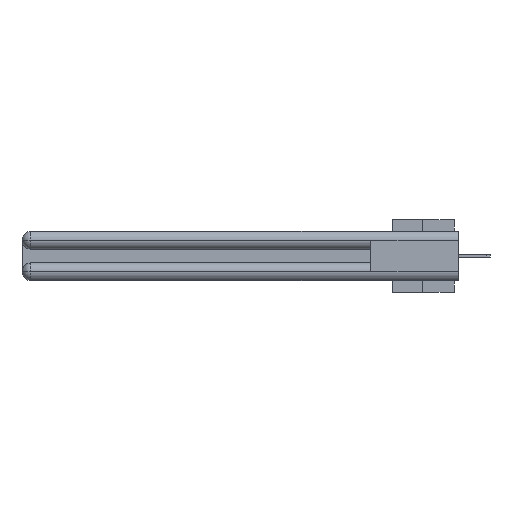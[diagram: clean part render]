
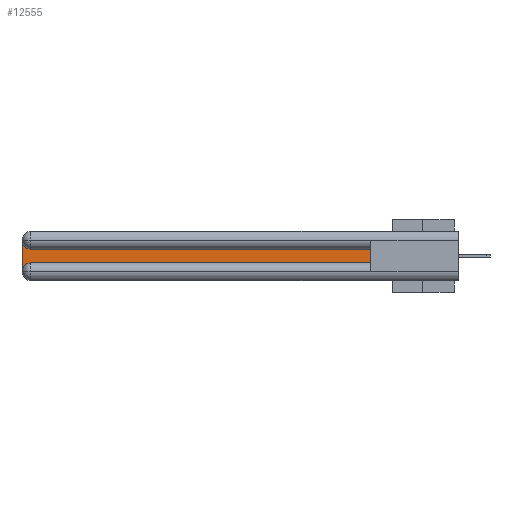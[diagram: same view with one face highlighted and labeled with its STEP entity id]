
A CAD part, left-side view. The second image highlights one B-rep face of the part: STEP entity #12555.
In plain terms, the highlighted planar face has unit normal (-1, 0, 0).
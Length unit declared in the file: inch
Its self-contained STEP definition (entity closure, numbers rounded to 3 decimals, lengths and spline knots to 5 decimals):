
#914 = CARTESIAN_POINT ( 'NONE',  ( 0.075, 3., -0.2175 ) ) ;
#1115 = DIRECTION ( 'NONE',  ( 0., 0., 1. ) ) ;
#2394 = ORIENTED_EDGE ( 'NONE', *, *, #29154, .T. ) ;
#2929 = EDGE_CURVE ( 'NONE', #7671, #6480, #18442, .T. ) ;
#2963 = DIRECTION ( 'NONE',  ( 1., 0., 0. ) ) ;
#3423 = VECTOR ( 'NONE', #14759, 39.37008 ) ;
#3445 = DIRECTION ( 'NONE',  ( 0., 0., -1. ) ) ;
#6480 = VERTEX_POINT ( 'NONE', #8833 ) ;
#7671 = VERTEX_POINT ( 'NONE', #31475 ) ;
#8169 = EDGE_CURVE ( 'NONE', #29907, #30754, #29712, .T. ) ;
#8724 = AXIS2_PLACEMENT_3D ( 'NONE', #18615, #2963, #21245 ) ;
#8833 = CARTESIAN_POINT ( 'NONE',  ( 0.075, 2.94, -0.2175 ) ) ;
#9157 = VECTOR ( 'NONE', #3445, 39.37008 ) ;
#9354 = CARTESIAN_POINT ( 'NONE',  ( 0.075, 0.6, -0.1225 ) ) ;
#9551 = LINE ( 'NONE', #30331, #3423 ) ;
#9962 = DIRECTION ( 'NONE',  ( 0., 0., -1. ) ) ;
#10489 = DIRECTION ( 'NONE',  ( 1., 0., 0. ) ) ;
#11056 = EDGE_CURVE ( 'NONE', #19192, #29907, #21841, .T. ) ;
#11895 = AXIS2_PLACEMENT_3D ( 'NONE', #26132, #10489, #28724 ) ;
#12555 = ADVANCED_FACE ( 'NONE', ( #16363 ), #22973, .F. ) ;
#12893 = ORIENTED_EDGE ( 'NONE', *, *, #11056, .T. ) ;
#14759 = DIRECTION ( 'NONE',  ( 0., -1., 0. ) ) ;
#14905 = VECTOR ( 'NONE', #27622, 39.37008 ) ;
#15080 = ORIENTED_EDGE ( 'NONE', *, *, #8169, .T. ) ;
#15100 = CARTESIAN_POINT ( 'NONE',  ( 0.075, 3., -0.0625 ) ) ;
#15238 = VERTEX_POINT ( 'NONE', #23461 ) ;
#16363 = FACE_OUTER_BOUND ( 'NONE', #23665, .T. ) ;
#16737 = EDGE_CURVE ( 'NONE', #30754, #7671, #23879, .T. ) ;
#16775 = CARTESIAN_POINT ( 'NONE',  ( 0.075, 0.6, -0.2175 ) ) ;
#16940 = EDGE_CURVE ( 'NONE', #6480, #15238, #9551, .T. ) ;
#18442 = CIRCLE ( 'NONE', #11895, 0.06 ) ;
#18615 = CARTESIAN_POINT ( 'NONE',  ( 0.075, 2.94, -0.0625 ) ) ;
#18657 = CARTESIAN_POINT ( 'NONE',  ( 0.075, 0.6, -0.1225 ) ) ;
#19192 = VERTEX_POINT ( 'NONE', #18657 ) ;
#19588 = CARTESIAN_POINT ( 'NONE',  ( 0.075, 2.94, -0.1225 ) ) ;
#21245 = DIRECTION ( 'NONE',  ( 0., 0., -1. ) ) ;
#21841 = LINE ( 'NONE', #9354, #14905 ) ;
#22973 = PLANE ( 'NONE',  #24128 ) ;
#23461 = CARTESIAN_POINT ( 'NONE',  ( 0.075, 0.6, -0.2175 ) ) ;
#23665 = EDGE_LOOP ( 'NONE', ( #12893, #15080, #30213, #33347, #26540, #2394 ) ) ;
#23879 = LINE ( 'NONE', #914, #9157 ) ;
#24128 = AXIS2_PLACEMENT_3D ( 'NONE', #25504, #25618, #9962 ) ;
#25504 = CARTESIAN_POINT ( 'NONE',  ( 0.075, 3., -0.1225 ) ) ;
#25618 = DIRECTION ( 'NONE',  ( 1., 0., 0. ) ) ;
#26132 = CARTESIAN_POINT ( 'NONE',  ( 0.075, 2.94, -0.2775 ) ) ;
#26540 = ORIENTED_EDGE ( 'NONE', *, *, #16940, .T. ) ;
#26787 = VECTOR ( 'NONE', #1115, 39.37008 ) ;
#27622 = DIRECTION ( 'NONE',  ( 0., 1., 0. ) ) ;
#28724 = DIRECTION ( 'NONE',  ( 0., 0., -1. ) ) ;
#29154 = EDGE_CURVE ( 'NONE', #15238, #19192, #31226, .T. ) ;
#29712 = CIRCLE ( 'NONE', #8724, 0.06 ) ;
#29907 = VERTEX_POINT ( 'NONE', #19588 ) ;
#30213 = ORIENTED_EDGE ( 'NONE', *, *, #16737, .T. ) ;
#30331 = CARTESIAN_POINT ( 'NONE',  ( 0.075, 0.6, -0.2175 ) ) ;
#30754 = VERTEX_POINT ( 'NONE', #15100 ) ;
#31226 = LINE ( 'NONE', #16775, #26787 ) ;
#31475 = CARTESIAN_POINT ( 'NONE',  ( 0.075, 3., -0.2775 ) ) ;
#33347 = ORIENTED_EDGE ( 'NONE', *, *, #2929, .T. ) ;
